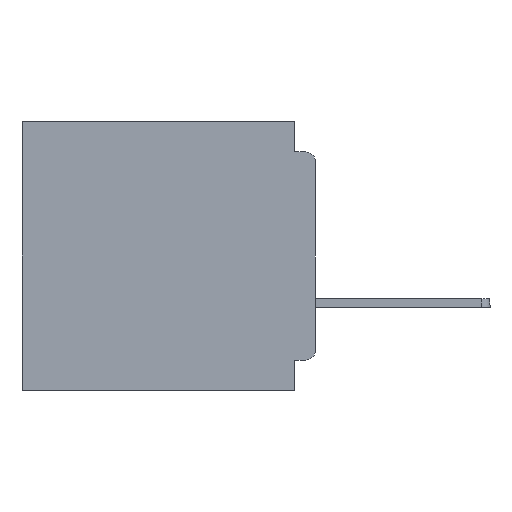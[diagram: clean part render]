
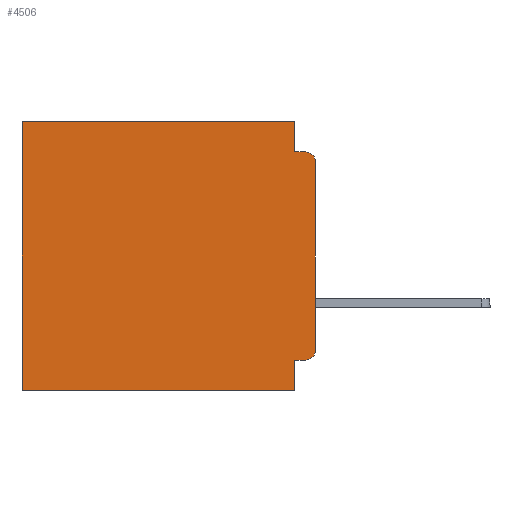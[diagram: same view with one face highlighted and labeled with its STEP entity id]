
A CAD part, left-side view. The second image highlights one B-rep face of the part: STEP entity #4506.
In plain terms, the highlighted planar face has unit normal (-1, 0, 0).
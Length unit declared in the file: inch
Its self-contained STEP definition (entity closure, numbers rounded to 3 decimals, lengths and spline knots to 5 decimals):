
#553 = VECTOR ( 'NONE', #32614, 39.37008 ) ;
#618 = DIRECTION ( 'NONE',  ( 0., 0., -1. ) ) ;
#759 = ORIENTED_EDGE ( 'NONE', *, *, #15937, .F. ) ;
#2045 = LINE ( 'NONE', #13472, #16992 ) ;
#2766 = VERTEX_POINT ( 'NONE', #39171 ) ;
#2868 = LINE ( 'NONE', #50477, #54450 ) ;
#3144 = CARTESIAN_POINT ( 'NONE',  ( 0.3, 0.437, -0.4 ) ) ;
#3185 = CARTESIAN_POINT ( 'NONE',  ( 0.3, 0.031, -0.4 ) ) ;
#4506 = ADVANCED_FACE ( 'NONE', ( #56524 ), #21832, .F. ) ;
#6242 = ORIENTED_EDGE ( 'NONE', *, *, #19083, .F. ) ;
#11753 = ORIENTED_EDGE ( 'NONE', *, *, #56759, .F. ) ;
#11763 = CARTESIAN_POINT ( 'NONE',  ( 0.3, 0., -0.4 ) ) ;
#13269 = CARTESIAN_POINT ( 'NONE',  ( 0.3, 0., -0.34 ) ) ;
#13472 = CARTESIAN_POINT ( 'NONE',  ( 0.3, 0., -0.045 ) ) ;
#15937 = EDGE_CURVE ( 'NONE', #33547, #47342, #45512, .T. ) ;
#16434 = ORIENTED_EDGE ( 'NONE', *, *, #57370, .F. ) ;
#16992 = VECTOR ( 'NONE', #53209, 39.37008 ) ;
#17603 = CARTESIAN_POINT ( 'NONE',  ( 0.3, 0.031, 0. ) ) ;
#18064 = DIRECTION ( 'NONE',  ( 0., 0., -1. ) ) ;
#19083 = EDGE_CURVE ( 'NONE', #47342, #48164, #26480, .T. ) ;
#19673 = VERTEX_POINT ( 'NONE', #29908 ) ;
#20425 = CIRCLE ( 'NONE', #52321, 0.015 ) ;
#20745 = DIRECTION ( 'NONE',  ( -1., 0., 0. ) ) ;
#21789 = VECTOR ( 'NONE', #40370, 39.37008 ) ;
#21832 = PLANE ( 'NONE',  #53551 ) ;
#21953 = EDGE_CURVE ( 'NONE', #48630, #61164, #30572, .T. ) ;
#24600 = DIRECTION ( 'NONE',  ( 0., 0., -1. ) ) ;
#25288 = CARTESIAN_POINT ( 'NONE',  ( 0.3, 0.031, 0. ) ) ;
#26480 = LINE ( 'NONE', #35393, #21789 ) ;
#26851 = DIRECTION ( 'NONE',  ( 0., 0., -1. ) ) ;
#28600 = CARTESIAN_POINT ( 'NONE',  ( 0.3, 0.015, -0.06 ) ) ;
#29908 = CARTESIAN_POINT ( 'NONE',  ( 0.3, 0., -0.06 ) ) ;
#30572 = LINE ( 'NONE', #38498, #43783 ) ;
#30598 = EDGE_CURVE ( 'NONE', #37749, #30921, #20425, .T. ) ;
#30921 = VERTEX_POINT ( 'NONE', #13269 ) ;
#32025 = EDGE_LOOP ( 'NONE', ( #16434, #56235, #45306, #11753, #33596, #53163, #6242, #759, #58107, #53230 ) ) ;
#32614 = DIRECTION ( 'NONE',  ( 0., 0., -1. ) ) ;
#33547 = VERTEX_POINT ( 'NONE', #53347 ) ;
#33596 = ORIENTED_EDGE ( 'NONE', *, *, #21953, .T. ) ;
#33613 = DIRECTION ( 'NONE',  ( 0., 0., -1. ) ) ;
#34611 = CARTESIAN_POINT ( 'NONE',  ( 0.3, 0.031, -0.4 ) ) ;
#35353 = LINE ( 'NONE', #3144, #47085 ) ;
#35393 = CARTESIAN_POINT ( 'NONE',  ( 0.3, 0., -0.4 ) ) ;
#35936 = CARTESIAN_POINT ( 'NONE',  ( 0.3, 0.437, 0. ) ) ;
#37009 = CARTESIAN_POINT ( 'NONE',  ( 0.3, 0., -0.355 ) ) ;
#37749 = VERTEX_POINT ( 'NONE', #63087 ) ;
#38498 = CARTESIAN_POINT ( 'NONE',  ( 0.3, 0., 0. ) ) ;
#39171 = CARTESIAN_POINT ( 'NONE',  ( 0.3, 0.031, -0.045 ) ) ;
#40370 = DIRECTION ( 'NONE',  ( 0., 1., 0. ) ) ;
#40406 = LINE ( 'NONE', #17603, #553 ) ;
#43783 = VECTOR ( 'NONE', #63454, 39.37008 ) ;
#44117 = LINE ( 'NONE', #37009, #57487 ) ;
#45306 = ORIENTED_EDGE ( 'NONE', *, *, #52048, .F. ) ;
#45512 = LINE ( 'NONE', #34611, #57273 ) ;
#47085 = VECTOR ( 'NONE', #18064, 39.37008 ) ;
#47342 = VERTEX_POINT ( 'NONE', #3185 ) ;
#47375 = CIRCLE ( 'NONE', #54754, 0.015 ) ;
#48031 = CARTESIAN_POINT ( 'NONE',  ( 0.3, 0.015, -0.045 ) ) ;
#48164 = VERTEX_POINT ( 'NONE', #59875 ) ;
#48630 = VERTEX_POINT ( 'NONE', #25288 ) ;
#50477 = CARTESIAN_POINT ( 'NONE',  ( 0.3, 0., -0.4 ) ) ;
#50635 = CARTESIAN_POINT ( 'NONE',  ( 0.3, 0.015, -0.34 ) ) ;
#51433 = VERTEX_POINT ( 'NONE', #48031 ) ;
#52048 = EDGE_CURVE ( 'NONE', #2766, #51433, #2045, .T. ) ;
#52321 = AXIS2_PLACEMENT_3D ( 'NONE', #50635, #20745, #55661 ) ;
#53163 = ORIENTED_EDGE ( 'NONE', *, *, #54877, .T. ) ;
#53209 = DIRECTION ( 'NONE',  ( 0., -1., 0. ) ) ;
#53230 = ORIENTED_EDGE ( 'NONE', *, *, #30598, .T. ) ;
#53347 = CARTESIAN_POINT ( 'NONE',  ( 0.3, 0.031, -0.355 ) ) ;
#53551 = AXIS2_PLACEMENT_3D ( 'NONE', #11763, #56734, #26851 ) ;
#54450 = VECTOR ( 'NONE', #618, 39.37008 ) ;
#54754 = AXIS2_PLACEMENT_3D ( 'NONE', #28600, #63542, #33613 ) ;
#54877 = EDGE_CURVE ( 'NONE', #61164, #48164, #35353, .T. ) ;
#55661 = DIRECTION ( 'NONE',  ( 0., 0., -1. ) ) ;
#56235 = ORIENTED_EDGE ( 'NONE', *, *, #57727, .T. ) ;
#56524 = FACE_OUTER_BOUND ( 'NONE', #32025, .T. ) ;
#56734 = DIRECTION ( 'NONE',  ( 1., 0., 0. ) ) ;
#56759 = EDGE_CURVE ( 'NONE', #48630, #2766, #40406, .T. ) ;
#57167 = DIRECTION ( 'NONE',  ( 0., 1., 0. ) ) ;
#57273 = VECTOR ( 'NONE', #24600, 39.37008 ) ;
#57370 = EDGE_CURVE ( 'NONE', #19673, #30921, #2868, .T. ) ;
#57487 = VECTOR ( 'NONE', #57167, 39.37008 ) ;
#57727 = EDGE_CURVE ( 'NONE', #19673, #51433, #47375, .T. ) ;
#58107 = ORIENTED_EDGE ( 'NONE', *, *, #58170, .F. ) ;
#58170 = EDGE_CURVE ( 'NONE', #37749, #33547, #44117, .T. ) ;
#59875 = CARTESIAN_POINT ( 'NONE',  ( 0.3, 0.437, -0.4 ) ) ;
#61164 = VERTEX_POINT ( 'NONE', #35936 ) ;
#63087 = CARTESIAN_POINT ( 'NONE',  ( 0.3, 0.015, -0.355 ) ) ;
#63454 = DIRECTION ( 'NONE',  ( 0., 1., 0. ) ) ;
#63542 = DIRECTION ( 'NONE',  ( -1., 0., 0. ) ) ;
